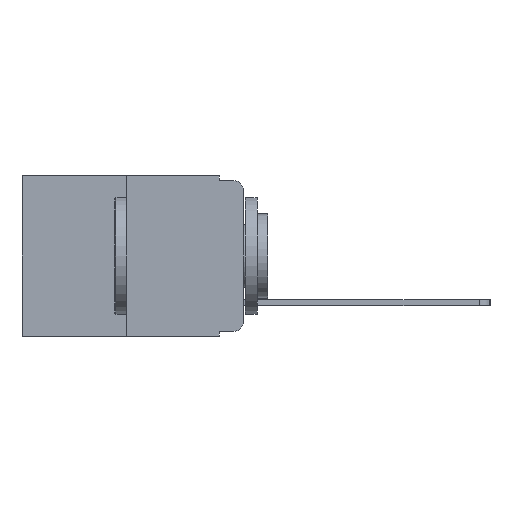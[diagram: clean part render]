
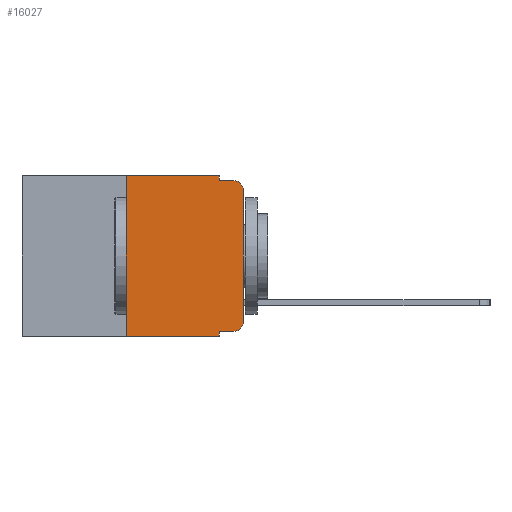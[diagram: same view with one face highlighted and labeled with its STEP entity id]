
A CAD part, left-side view. The second image highlights one B-rep face of the part: STEP entity #16027.
In plain terms, the highlighted planar face has unit normal (-1, 0, 0).
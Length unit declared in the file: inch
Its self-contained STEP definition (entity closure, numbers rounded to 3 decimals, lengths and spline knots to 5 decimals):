
#239 = LINE ( 'NONE', #13622, #16305 ) ;
#415 = CARTESIAN_POINT ( 'NONE',  ( 0., 0.051, -0.01 ) ) ;
#530 = VECTOR ( 'NONE', #4151, 39.37008 ) ;
#612 = AXIS2_PLACEMENT_3D ( 'NONE', #10230, #13301, #4042 ) ;
#1391 = CARTESIAN_POINT ( 'NONE',  ( 0., 0.25, 0. ) ) ;
#1522 = CARTESIAN_POINT ( 'NONE',  ( 0., 0., 0. ) ) ;
#1659 = ORIENTED_EDGE ( 'NONE', *, *, #16621, .F. ) ;
#1742 = ORIENTED_EDGE ( 'NONE', *, *, #18801, .F. ) ;
#2047 = ORIENTED_EDGE ( 'NONE', *, *, #6751, .T. ) ;
#2139 = VERTEX_POINT ( 'NONE', #1391 ) ;
#2503 = CARTESIAN_POINT ( 'NONE',  ( 0., 0.051, -0.333 ) ) ;
#2660 = CARTESIAN_POINT ( 'NONE',  ( 0., 0.25, -0.343 ) ) ;
#2771 = ORIENTED_EDGE ( 'NONE', *, *, #16187, .F. ) ;
#3003 = CARTESIAN_POINT ( 'NONE',  ( 0., 0.02, -0.03 ) ) ;
#3229 = ORIENTED_EDGE ( 'NONE', *, *, #4208, .T. ) ;
#3260 = ORIENTED_EDGE ( 'NONE', *, *, #5301, .T. ) ;
#4042 = DIRECTION ( 'NONE',  ( 0., 0., -1. ) ) ;
#4151 = DIRECTION ( 'NONE',  ( 0., -1., 0. ) ) ;
#4208 = EDGE_CURVE ( 'NONE', #12407, #8530, #8085, .T. ) ;
#4393 = ORIENTED_EDGE ( 'NONE', *, *, #10820, .F. ) ;
#4618 = DIRECTION ( 'NONE',  ( 0., 0., -1. ) ) ;
#4974 = CARTESIAN_POINT ( 'NONE',  ( 0., 0., -0.313 ) ) ;
#5301 = EDGE_CURVE ( 'NONE', #8530, #9297, #16728, .T. ) ;
#5448 = CARTESIAN_POINT ( 'NONE',  ( 0., 0.473, -0.343 ) ) ;
#6197 = VECTOR ( 'NONE', #14598, 39.37008 ) ;
#6751 = EDGE_CURVE ( 'NONE', #14248, #11100, #10262, .T. ) ;
#6825 = CARTESIAN_POINT ( 'NONE',  ( 0., 0.02, -0.313 ) ) ;
#7506 = FACE_OUTER_BOUND ( 'NONE', #16036, .T. ) ;
#7971 = VECTOR ( 'NONE', #17897, 39.37008 ) ;
#8085 = LINE ( 'NONE', #2503, #12615 ) ;
#8330 = DIRECTION ( 'NONE',  ( 0., 0., -1. ) ) ;
#8515 = VERTEX_POINT ( 'NONE', #415 ) ;
#8530 = VERTEX_POINT ( 'NONE', #17491 ) ;
#8735 = CARTESIAN_POINT ( 'NONE',  ( 0., 0.051, -0.333 ) ) ;
#8766 = CARTESIAN_POINT ( 'NONE',  ( 0., 0.473, 0. ) ) ;
#9297 = VERTEX_POINT ( 'NONE', #4974 ) ;
#10162 = ORIENTED_EDGE ( 'NONE', *, *, #14914, .F. ) ;
#10230 = CARTESIAN_POINT ( 'NONE',  ( 0., 0.473, 0. ) ) ;
#10262 = LINE ( 'NONE', #5448, #6197 ) ;
#10465 = CARTESIAN_POINT ( 'NONE',  ( 0., 0.051, 0. ) ) ;
#10811 = DIRECTION ( 'NONE',  ( 0., 0., 1. ) ) ;
#10820 = EDGE_CURVE ( 'NONE', #16669, #8515, #12033, .T. ) ;
#11014 = LINE ( 'NONE', #14443, #14592 ) ;
#11100 = VERTEX_POINT ( 'NONE', #12493 ) ;
#11820 = CARTESIAN_POINT ( 'NONE',  ( 0., 0.02, -0.01 ) ) ;
#12017 = AXIS2_PLACEMENT_3D ( 'NONE', #6825, #17442, #8330 ) ;
#12033 = LINE ( 'NONE', #16416, #7971 ) ;
#12407 = VERTEX_POINT ( 'NONE', #8735 ) ;
#12493 = CARTESIAN_POINT ( 'NONE',  ( 0., 0.051, -0.343 ) ) ;
#12531 = LINE ( 'NONE', #13396, #530 ) ;
#12615 = VECTOR ( 'NONE', #19232, 39.37008 ) ;
#12730 = LINE ( 'NONE', #8766, #15814 ) ;
#12984 = LINE ( 'NONE', #1522, #16063 ) ;
#12988 = VERTEX_POINT ( 'NONE', #11820 ) ;
#13232 = PLANE ( 'NONE',  #612 ) ;
#13301 = DIRECTION ( 'NONE',  ( 1., 0., 0. ) ) ;
#13396 = CARTESIAN_POINT ( 'NONE',  ( 0., 0.051, -0.01 ) ) ;
#13426 = ORIENTED_EDGE ( 'NONE', *, *, #17911, .T. ) ;
#13450 = ORIENTED_EDGE ( 'NONE', *, *, #13778, .T. ) ;
#13622 = CARTESIAN_POINT ( 'NONE',  ( 0., 0.051, 0. ) ) ;
#13696 = CIRCLE ( 'NONE', #13952, 0.02 ) ;
#13778 = EDGE_CURVE ( 'NONE', #9297, #17282, #12984, .T. ) ;
#13817 = DIRECTION ( 'NONE',  ( -1., 0., 0. ) ) ;
#13952 = AXIS2_PLACEMENT_3D ( 'NONE', #3003, #13817, #4618 ) ;
#14248 = VERTEX_POINT ( 'NONE', #2660 ) ;
#14443 = CARTESIAN_POINT ( 'NONE',  ( 0., 0.25, 0. ) ) ;
#14592 = VECTOR ( 'NONE', #15965, 39.37008 ) ;
#14598 = DIRECTION ( 'NONE',  ( 0., -1., 0. ) ) ;
#14914 = EDGE_CURVE ( 'NONE', #8515, #12988, #12531, .T. ) ;
#14922 = DIRECTION ( 'NONE',  ( 0., -1., 0. ) ) ;
#15814 = VECTOR ( 'NONE', #14922, 39.37008 ) ;
#15965 = DIRECTION ( 'NONE',  ( 0., 0., 1. ) ) ;
#16027 = ADVANCED_FACE ( 'NONE', ( #7506 ), #13232, .F. ) ;
#16036 = EDGE_LOOP ( 'NONE', ( #13450, #13426, #10162, #4393, #1659, #1742, #2047, #2771, #3229, #3260 ) ) ;
#16063 = VECTOR ( 'NONE', #10811, 39.37008 ) ;
#16187 = EDGE_CURVE ( 'NONE', #12407, #11100, #239, .T. ) ;
#16305 = VECTOR ( 'NONE', #16663, 39.37008 ) ;
#16416 = CARTESIAN_POINT ( 'NONE',  ( 0., 0.051, 0. ) ) ;
#16621 = EDGE_CURVE ( 'NONE', #2139, #16669, #12730, .T. ) ;
#16663 = DIRECTION ( 'NONE',  ( 0., 0., -1. ) ) ;
#16669 = VERTEX_POINT ( 'NONE', #10465 ) ;
#16728 = CIRCLE ( 'NONE', #12017, 0.02 ) ;
#17282 = VERTEX_POINT ( 'NONE', #19604 ) ;
#17442 = DIRECTION ( 'NONE',  ( -1., 0., 0. ) ) ;
#17491 = CARTESIAN_POINT ( 'NONE',  ( 0., 0.02, -0.333 ) ) ;
#17897 = DIRECTION ( 'NONE',  ( 0., 0., -1. ) ) ;
#17911 = EDGE_CURVE ( 'NONE', #17282, #12988, #13696, .T. ) ;
#18801 = EDGE_CURVE ( 'NONE', #14248, #2139, #11014, .T. ) ;
#19232 = DIRECTION ( 'NONE',  ( 0., -1., 0. ) ) ;
#19604 = CARTESIAN_POINT ( 'NONE',  ( 0., 0., -0.03 ) ) ;
